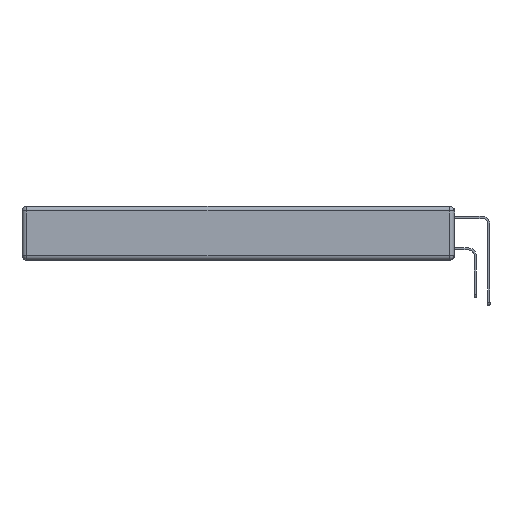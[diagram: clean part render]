
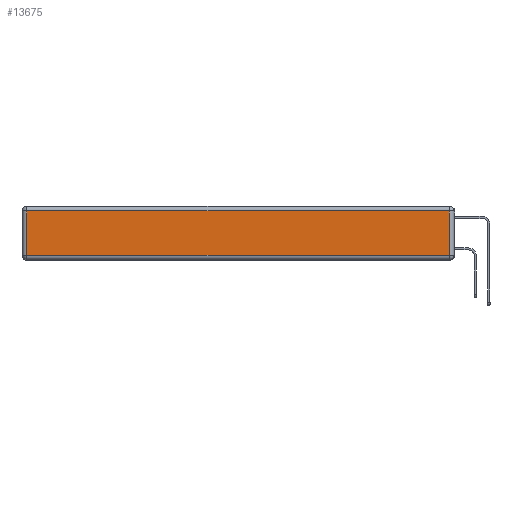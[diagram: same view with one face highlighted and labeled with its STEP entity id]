
A CAD part, left-side view. The second image highlights one B-rep face of the part: STEP entity #13675.
In plain terms, the highlighted planar face has unit normal (-1, 0, 0).
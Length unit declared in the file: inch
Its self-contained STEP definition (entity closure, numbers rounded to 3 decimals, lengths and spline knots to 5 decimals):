
#101 = ORIENTED_EDGE ( 'NONE', *, *, #1766, .T. ) ;
#606 = CARTESIAN_POINT ( 'NONE',  ( 0., 0., -0.343 ) ) ;
#622 = CARTESIAN_POINT ( 'NONE',  ( 0., 0., -0.313 ) ) ;
#1425 = CARTESIAN_POINT ( 'NONE',  ( 0., 2.72, -0.03 ) ) ;
#1505 = VERTEX_POINT ( 'NONE', #16029 ) ;
#1766 = EDGE_CURVE ( 'NONE', #5904, #11711, #9331, .T. ) ;
#2231 = VECTOR ( 'NONE', #16558, 39.37008 ) ;
#2294 = DIRECTION ( 'NONE',  ( 0., -1., 0. ) ) ;
#2529 = ORIENTED_EDGE ( 'NONE', *, *, #5664, .T. ) ;
#2990 = EDGE_CURVE ( 'NONE', #1505, #5904, #18560, .T. ) ;
#4050 = VECTOR ( 'NONE', #13939, 39.37008 ) ;
#5115 = DIRECTION ( 'NONE',  ( 0., 0., 1. ) ) ;
#5210 = PLANE ( 'NONE',  #19297 ) ;
#5590 = LINE ( 'NONE', #10474, #14738 ) ;
#5664 = EDGE_CURVE ( 'NONE', #11711, #6062, #6069, .T. ) ;
#5904 = VERTEX_POINT ( 'NONE', #14558 ) ;
#6062 = VERTEX_POINT ( 'NONE', #1425 ) ;
#6069 = LINE ( 'NONE', #9204, #2231 ) ;
#6584 = DIRECTION ( 'NONE',  ( -1., 0., 0. ) ) ;
#6889 = EDGE_CURVE ( 'NONE', #6062, #1505, #5590, .T. ) ;
#9204 = CARTESIAN_POINT ( 'NONE',  ( 0., 2.75, -0.03 ) ) ;
#9331 = LINE ( 'NONE', #15322, #4050 ) ;
#9503 = CARTESIAN_POINT ( 'NONE',  ( 0., 0.03, -0.03 ) ) ;
#10024 = ORIENTED_EDGE ( 'NONE', *, *, #6889, .T. ) ;
#10474 = CARTESIAN_POINT ( 'NONE',  ( 0., 2.72, -0.343 ) ) ;
#11011 = EDGE_LOOP ( 'NONE', ( #17006, #101, #2529, #10024 ) ) ;
#11711 = VERTEX_POINT ( 'NONE', #9503 ) ;
#13239 = DIRECTION ( 'NONE',  ( 0., 0., -1. ) ) ;
#13675 = ADVANCED_FACE ( 'NONE', ( #18542 ), #5210, .T. ) ;
#13939 = DIRECTION ( 'NONE',  ( 0., 0., 1. ) ) ;
#14042 = VECTOR ( 'NONE', #2294, 39.37008 ) ;
#14558 = CARTESIAN_POINT ( 'NONE',  ( 0., 0.03, -0.313 ) ) ;
#14738 = VECTOR ( 'NONE', #13239, 39.37008 ) ;
#15322 = CARTESIAN_POINT ( 'NONE',  ( 0., 0.03, -0.343 ) ) ;
#16029 = CARTESIAN_POINT ( 'NONE',  ( 0., 2.72, -0.313 ) ) ;
#16558 = DIRECTION ( 'NONE',  ( 0., 1., 0. ) ) ;
#17006 = ORIENTED_EDGE ( 'NONE', *, *, #2990, .T. ) ;
#18542 = FACE_OUTER_BOUND ( 'NONE', #11011, .T. ) ;
#18560 = LINE ( 'NONE', #622, #14042 ) ;
#19297 = AXIS2_PLACEMENT_3D ( 'NONE', #606, #6584, #5115 ) ;
